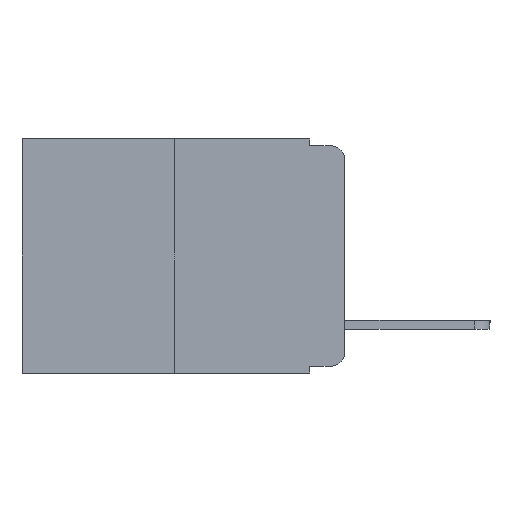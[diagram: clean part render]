
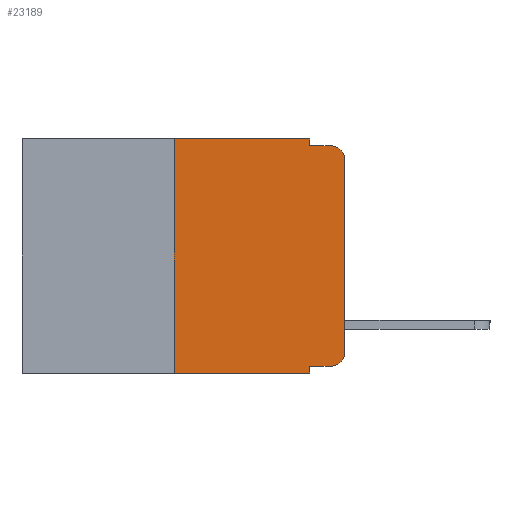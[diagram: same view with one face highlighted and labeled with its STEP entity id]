
A CAD part, left-side view. The second image highlights one B-rep face of the part: STEP entity #23189.
In plain terms, the highlighted planar face has unit normal (-1, 0, 0).
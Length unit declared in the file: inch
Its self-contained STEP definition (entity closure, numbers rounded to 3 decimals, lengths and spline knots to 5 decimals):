
#66 = VERTEX_POINT ( 'NONE', #11829 ) ;
#1681 = DIRECTION ( 'NONE',  ( 0., -1., 0. ) ) ;
#3255 = LINE ( 'NONE', #11040, #8847 ) ;
#3659 = LINE ( 'NONE', #11562, #23866 ) ;
#3695 = ORIENTED_EDGE ( 'NONE', *, *, #14461, .F. ) ;
#3970 = VERTEX_POINT ( 'NONE', #5493 ) ;
#4026 = DIRECTION ( 'NONE',  ( 1., 0., 0. ) ) ;
#4459 = CARTESIAN_POINT ( 'NONE',  ( 0., 0.473, -0.343 ) ) ;
#4638 = CARTESIAN_POINT ( 'NONE',  ( 0., 0.051, -0.01 ) ) ;
#4775 = LINE ( 'NONE', #8810, #10301 ) ;
#4896 = EDGE_LOOP ( 'NONE', ( #10602, #16517, #19820, #9466, #3695, #13023, #7289, #18897, #19508, #15239 ) ) ;
#5493 = CARTESIAN_POINT ( 'NONE',  ( 0., 0., -0.313 ) ) ;
#5898 = CARTESIAN_POINT ( 'NONE',  ( 0., 0.02, -0.03 ) ) ;
#6109 = VECTOR ( 'NONE', #23884, 39.37008 ) ;
#6462 = CARTESIAN_POINT ( 'NONE',  ( 0., 0.25, 0. ) ) ;
#6523 = VERTEX_POINT ( 'NONE', #17096 ) ;
#6770 = EDGE_CURVE ( 'NONE', #19991, #24155, #24700, .T. ) ;
#7264 = EDGE_CURVE ( 'NONE', #6523, #24155, #18342, .T. ) ;
#7289 = ORIENTED_EDGE ( 'NONE', *, *, #6770, .T. ) ;
#7323 = DIRECTION ( 'NONE',  ( 0., 0., -1. ) ) ;
#7834 = EDGE_CURVE ( 'NONE', #8069, #3970, #16540, .T. ) ;
#7859 = EDGE_CURVE ( 'NONE', #3970, #25081, #4775, .T. ) ;
#8069 = VERTEX_POINT ( 'NONE', #8620 ) ;
#8620 = CARTESIAN_POINT ( 'NONE',  ( 0., 0.02, -0.333 ) ) ;
#8810 = CARTESIAN_POINT ( 'NONE',  ( 0., 0., 0. ) ) ;
#8847 = VECTOR ( 'NONE', #11547, 39.37008 ) ;
#9466 = ORIENTED_EDGE ( 'NONE', *, *, #19129, .F. ) ;
#9853 = FACE_OUTER_BOUND ( 'NONE', #4896, .T. ) ;
#10301 = VECTOR ( 'NONE', #16726, 39.37008 ) ;
#10471 = LINE ( 'NONE', #4638, #6109 ) ;
#10573 = LINE ( 'NONE', #18523, #17327 ) ;
#10602 = ORIENTED_EDGE ( 'NONE', *, *, #7859, .T. ) ;
#10840 = DIRECTION ( 'NONE',  ( 0., 0., 1. ) ) ;
#10946 = VERTEX_POINT ( 'NONE', #19603 ) ;
#11040 = CARTESIAN_POINT ( 'NONE',  ( 0., 0.473, 0. ) ) ;
#11547 = DIRECTION ( 'NONE',  ( 0., -1., 0. ) ) ;
#11562 = CARTESIAN_POINT ( 'NONE',  ( 0., 0.051, -0.333 ) ) ;
#11829 = CARTESIAN_POINT ( 'NONE',  ( 0., 0.02, -0.01 ) ) ;
#12255 = CARTESIAN_POINT ( 'NONE',  ( 0., 0.25, -0.343 ) ) ;
#12993 = CARTESIAN_POINT ( 'NONE',  ( 0., 0.051, -0.01 ) ) ;
#13023 = ORIENTED_EDGE ( 'NONE', *, *, #20129, .F. ) ;
#13053 = CARTESIAN_POINT ( 'NONE',  ( 0., 0.02, -0.313 ) ) ;
#14461 = EDGE_CURVE ( 'NONE', #19707, #10946, #3255, .T. ) ;
#14871 = AXIS2_PLACEMENT_3D ( 'NONE', #21830, #4026, #19889 ) ;
#15099 = CARTESIAN_POINT ( 'NONE',  ( 0., 0.051, 0. ) ) ;
#15138 = DIRECTION ( 'NONE',  ( 0., 0., -1. ) ) ;
#15239 = ORIENTED_EDGE ( 'NONE', *, *, #7834, .T. ) ;
#15728 = LINE ( 'NONE', #15099, #16433 ) ;
#15878 = DIRECTION ( 'NONE',  ( 0., 0., -1. ) ) ;
#16024 = CARTESIAN_POINT ( 'NONE',  ( 0., 0.051, -0.343 ) ) ;
#16244 = DIRECTION ( 'NONE',  ( 0., 0., -1. ) ) ;
#16433 = VECTOR ( 'NONE', #7323, 39.37008 ) ;
#16517 = ORIENTED_EDGE ( 'NONE', *, *, #25177, .T. ) ;
#16540 = CIRCLE ( 'NONE', #17805, 0.02 ) ;
#16726 = DIRECTION ( 'NONE',  ( 0., 0., 1. ) ) ;
#17096 = CARTESIAN_POINT ( 'NONE',  ( 0., 0.051, -0.333 ) ) ;
#17327 = VECTOR ( 'NONE', #10840, 39.37008 ) ;
#17805 = AXIS2_PLACEMENT_3D ( 'NONE', #13053, #22969, #15138 ) ;
#17939 = EDGE_CURVE ( 'NONE', #6523, #8069, #3659, .T. ) ;
#18342 = LINE ( 'NONE', #24296, #25590 ) ;
#18523 = CARTESIAN_POINT ( 'NONE',  ( 0., 0.25, 0. ) ) ;
#18755 = DIRECTION ( 'NONE',  ( 0., -1., 0. ) ) ;
#18897 = ORIENTED_EDGE ( 'NONE', *, *, #7264, .F. ) ;
#19129 = EDGE_CURVE ( 'NONE', #10946, #24246, #15728, .T. ) ;
#19508 = ORIENTED_EDGE ( 'NONE', *, *, #17939, .T. ) ;
#19559 = DIRECTION ( 'NONE',  ( -1., 0., 0. ) ) ;
#19603 = CARTESIAN_POINT ( 'NONE',  ( 0., 0.051, 0. ) ) ;
#19677 = EDGE_CURVE ( 'NONE', #24246, #66, #10471, .T. ) ;
#19707 = VERTEX_POINT ( 'NONE', #6462 ) ;
#19820 = ORIENTED_EDGE ( 'NONE', *, *, #19677, .F. ) ;
#19889 = DIRECTION ( 'NONE',  ( 0., 0., -1. ) ) ;
#19991 = VERTEX_POINT ( 'NONE', #12255 ) ;
#20129 = EDGE_CURVE ( 'NONE', #19991, #19707, #10573, .T. ) ;
#20612 = CIRCLE ( 'NONE', #21038, 0.02 ) ;
#21038 = AXIS2_PLACEMENT_3D ( 'NONE', #5898, #19559, #15878 ) ;
#21242 = CARTESIAN_POINT ( 'NONE',  ( 0., 0., -0.03 ) ) ;
#21830 = CARTESIAN_POINT ( 'NONE',  ( 0., 0.473, 0. ) ) ;
#22969 = DIRECTION ( 'NONE',  ( -1., 0., 0. ) ) ;
#23189 = ADVANCED_FACE ( 'NONE', ( #9853 ), #23761, .F. ) ;
#23761 = PLANE ( 'NONE',  #14871 ) ;
#23866 = VECTOR ( 'NONE', #1681, 39.37008 ) ;
#23884 = DIRECTION ( 'NONE',  ( 0., -1., 0. ) ) ;
#24155 = VERTEX_POINT ( 'NONE', #16024 ) ;
#24246 = VERTEX_POINT ( 'NONE', #12993 ) ;
#24285 = VECTOR ( 'NONE', #18755, 39.37008 ) ;
#24296 = CARTESIAN_POINT ( 'NONE',  ( 0., 0.051, 0. ) ) ;
#24700 = LINE ( 'NONE', #4459, #24285 ) ;
#25081 = VERTEX_POINT ( 'NONE', #21242 ) ;
#25177 = EDGE_CURVE ( 'NONE', #25081, #66, #20612, .T. ) ;
#25590 = VECTOR ( 'NONE', #16244, 39.37008 ) ;
